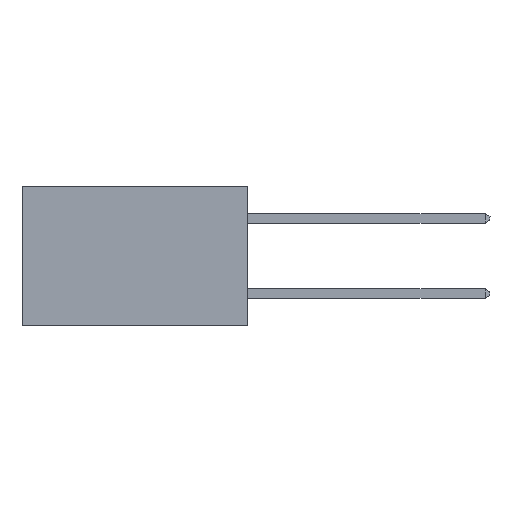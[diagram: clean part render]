
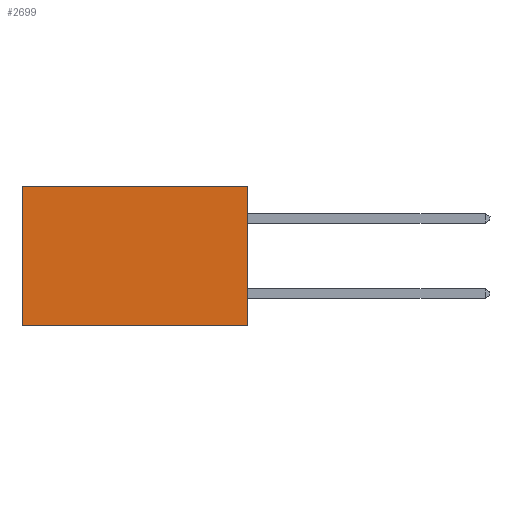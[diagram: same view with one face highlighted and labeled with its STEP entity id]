
A CAD part, left-side view. The second image highlights one B-rep face of the part: STEP entity #2699.
In plain terms, the highlighted planar face has unit normal (-1, 0, 0).
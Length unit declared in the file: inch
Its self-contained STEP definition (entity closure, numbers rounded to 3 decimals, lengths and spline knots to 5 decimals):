
#113 = ORIENTED_EDGE ( 'NONE', *, *, #4077, .T. ) ;
#203 = CARTESIAN_POINT ( 'NONE',  ( 0.2615, 0., 0. ) ) ;
#721 = CARTESIAN_POINT ( 'NONE',  ( 0.2615, 0., -0.37 ) ) ;
#1740 = EDGE_CURVE ( 'NONE', #8031, #6570, #2726, .T. ) ;
#1844 = CARTESIAN_POINT ( 'NONE',  ( 0.2615, 0., -0.37 ) ) ;
#2191 = VERTEX_POINT ( 'NONE', #2399 ) ;
#2399 = CARTESIAN_POINT ( 'NONE',  ( 0.2615, 0.6, -0.37 ) ) ;
#2403 = DIRECTION ( 'NONE',  ( 0., 1., 0. ) ) ;
#2475 = VECTOR ( 'NONE', #2403, 39.37008 ) ;
#2618 = DIRECTION ( 'NONE',  ( 0., 1., 0. ) ) ;
#2699 = ADVANCED_FACE ( 'NONE', ( #2896 ), #7242, .F. ) ;
#2726 = LINE ( 'NONE', #3272, #5805 ) ;
#2791 = VERTEX_POINT ( 'NONE', #7199 ) ;
#2896 = FACE_OUTER_BOUND ( 'NONE', #3603, .T. ) ;
#3272 = CARTESIAN_POINT ( 'NONE',  ( 0.2615, 0., -0.37 ) ) ;
#3341 = LINE ( 'NONE', #1844, #5033 ) ;
#3391 = ORIENTED_EDGE ( 'NONE', *, *, #6014, .F. ) ;
#3603 = EDGE_LOOP ( 'NONE', ( #6803, #3391, #8109, #113 ) ) ;
#3605 = VECTOR ( 'NONE', #7616, 39.37008 ) ;
#4077 = EDGE_CURVE ( 'NONE', #8031, #2791, #6040, .T. ) ;
#4450 = DIRECTION ( 'NONE',  ( 1., 0., 0. ) ) ;
#4459 = CARTESIAN_POINT ( 'NONE',  ( 0.2615, 0., -0.37 ) ) ;
#4574 = DIRECTION ( 'NONE',  ( 0., 0., -1. ) ) ;
#4739 = LINE ( 'NONE', #6834, #3605 ) ;
#5033 = VECTOR ( 'NONE', #2618, 39.37008 ) ;
#5805 = VECTOR ( 'NONE', #4574, 39.37008 ) ;
#6014 = EDGE_CURVE ( 'NONE', #6570, #2191, #3341, .T. ) ;
#6040 = LINE ( 'NONE', #203, #2475 ) ;
#6519 = CARTESIAN_POINT ( 'NONE',  ( 0.2615, 0., 0. ) ) ;
#6570 = VERTEX_POINT ( 'NONE', #4459 ) ;
#6803 = ORIENTED_EDGE ( 'NONE', *, *, #7323, .T. ) ;
#6834 = CARTESIAN_POINT ( 'NONE',  ( 0.2615, 0.6, -0.37 ) ) ;
#7199 = CARTESIAN_POINT ( 'NONE',  ( 0.2615, 0.6, 0. ) ) ;
#7242 = PLANE ( 'NONE',  #8993 ) ;
#7323 = EDGE_CURVE ( 'NONE', #2791, #2191, #4739, .T. ) ;
#7616 = DIRECTION ( 'NONE',  ( 0., 0., -1. ) ) ;
#8031 = VERTEX_POINT ( 'NONE', #6519 ) ;
#8109 = ORIENTED_EDGE ( 'NONE', *, *, #1740, .F. ) ;
#8749 = DIRECTION ( 'NONE',  ( 0., 0., -1. ) ) ;
#8993 = AXIS2_PLACEMENT_3D ( 'NONE', #721, #4450, #8749 ) ;
